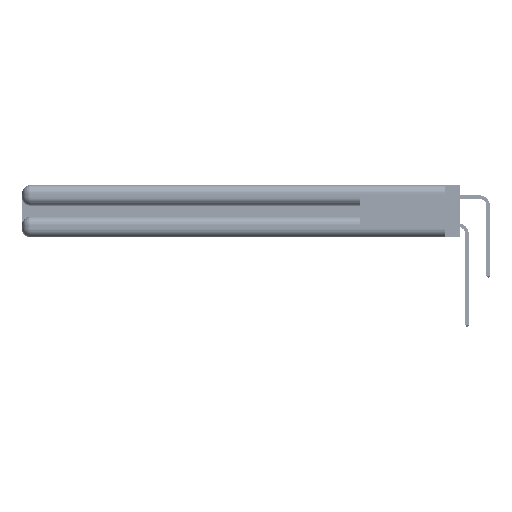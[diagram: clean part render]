
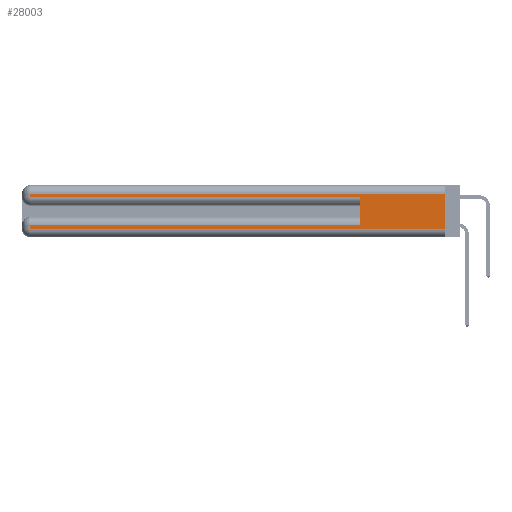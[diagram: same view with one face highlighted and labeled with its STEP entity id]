
A CAD part, left-side view. The second image highlights one B-rep face of the part: STEP entity #28003.
In plain terms, the highlighted planar face has unit normal (-1, 0, 0).
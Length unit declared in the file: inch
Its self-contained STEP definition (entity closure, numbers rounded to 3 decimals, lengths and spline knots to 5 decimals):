
#522 = CARTESIAN_POINT ( 'NONE',  ( 0., 0., 0.37 ) ) ;
#629 = CARTESIAN_POINT ( 'NONE',  ( 0., 0., 0.085 ) ) ;
#1703 = ORIENTED_EDGE ( 'NONE', *, *, #43113, .F. ) ;
#3313 = LINE ( 'NONE', #629, #13227 ) ;
#3759 = ORIENTED_EDGE ( 'NONE', *, *, #35805, .T. ) ;
#3783 = FACE_OUTER_BOUND ( 'NONE', #12405, .T. ) ;
#3843 = EDGE_CURVE ( 'NONE', #17330, #5140, #22326, .T. ) ;
#5140 = VERTEX_POINT ( 'NONE', #45637 ) ;
#5736 = ORIENTED_EDGE ( 'NONE', *, *, #45919, .T. ) ;
#9305 = PLANE ( 'NONE',  #9747 ) ;
#9747 = AXIS2_PLACEMENT_3D ( 'NONE', #522, #17726, #46899 ) ;
#9987 = CARTESIAN_POINT ( 'NONE',  ( 0., 2.94, 0.37 ) ) ;
#10115 = CARTESIAN_POINT ( 'NONE',  ( 0., 0., 0.285 ) ) ;
#11299 = VECTOR ( 'NONE', #47734, 39.37008 ) ;
#11415 = LINE ( 'NONE', #25395, #32263 ) ;
#11681 = EDGE_CURVE ( 'NONE', #12566, #37093, #11415, .T. ) ;
#12405 = EDGE_LOOP ( 'NONE', ( #1703, #5736, #18234, #43026, #13668, #35899, #3759, #41088 ) ) ;
#12566 = VERTEX_POINT ( 'NONE', #14197 ) ;
#13227 = VECTOR ( 'NONE', #34418, 39.37008 ) ;
#13397 = EDGE_CURVE ( 'NONE', #28808, #53611, #3313, .T. ) ;
#13668 = ORIENTED_EDGE ( 'NONE', *, *, #38563, .F. ) ;
#14197 = CARTESIAN_POINT ( 'NONE',  ( 0., 2.94, 0.06 ) ) ;
#14867 = CARTESIAN_POINT ( 'NONE',  ( 0., 2.94, 0.085 ) ) ;
#16920 = DIRECTION ( 'NONE',  ( 0., 0., 1. ) ) ;
#17330 = VERTEX_POINT ( 'NONE', #19297 ) ;
#17409 = VECTOR ( 'NONE', #16920, 39.37008 ) ;
#17726 = DIRECTION ( 'NONE',  ( 1., 0., 0. ) ) ;
#18234 = ORIENTED_EDGE ( 'NONE', *, *, #23566, .T. ) ;
#19297 = CARTESIAN_POINT ( 'NONE',  ( 0., 2.94, 0.285 ) ) ;
#22326 = LINE ( 'NONE', #10115, #52970 ) ;
#22356 = LINE ( 'NONE', #22564, #11299 ) ;
#22564 = CARTESIAN_POINT ( 'NONE',  ( 0., 0., 0.31 ) ) ;
#22972 = LINE ( 'NONE', #39058, #43829 ) ;
#23566 = EDGE_CURVE ( 'NONE', #33350, #17330, #24804, .T. ) ;
#24804 = LINE ( 'NONE', #9987, #26114 ) ;
#25395 = CARTESIAN_POINT ( 'NONE',  ( 0., 0., 0.06 ) ) ;
#26114 = VECTOR ( 'NONE', #39190, 39.37008 ) ;
#28003 = ADVANCED_FACE ( 'NONE', ( #3783 ), #9305, .F. ) ;
#28507 = LINE ( 'NONE', #46086, #17409 ) ;
#28808 = VERTEX_POINT ( 'NONE', #51543 ) ;
#29594 = DIRECTION ( 'NONE',  ( 0., -1., 0. ) ) ;
#30323 = CARTESIAN_POINT ( 'NONE',  ( 0., 2.94, 0.31 ) ) ;
#31305 = CARTESIAN_POINT ( 'NONE',  ( 0., 0., 0.06 ) ) ;
#32263 = VECTOR ( 'NONE', #29594, 39.37008 ) ;
#33282 = LINE ( 'NONE', #41391, #43045 ) ;
#33350 = VERTEX_POINT ( 'NONE', #30323 ) ;
#34418 = DIRECTION ( 'NONE',  ( 0., 1., 0. ) ) ;
#34880 = DIRECTION ( 'NONE',  ( 0., 0., -1. ) ) ;
#35805 = EDGE_CURVE ( 'NONE', #53611, #12566, #22972, .T. ) ;
#35899 = ORIENTED_EDGE ( 'NONE', *, *, #13397, .T. ) ;
#37093 = VERTEX_POINT ( 'NONE', #31305 ) ;
#38563 = EDGE_CURVE ( 'NONE', #28808, #5140, #28507, .T. ) ;
#39058 = CARTESIAN_POINT ( 'NONE',  ( 0., 2.94, 0.37 ) ) ;
#39190 = DIRECTION ( 'NONE',  ( 0., 0., -1. ) ) ;
#41088 = ORIENTED_EDGE ( 'NONE', *, *, #11681, .T. ) ;
#41391 = CARTESIAN_POINT ( 'NONE',  ( 0., 0., 0.37 ) ) ;
#43026 = ORIENTED_EDGE ( 'NONE', *, *, #3843, .T. ) ;
#43045 = VECTOR ( 'NONE', #45584, 39.37008 ) ;
#43113 = EDGE_CURVE ( 'NONE', #44246, #37093, #33282, .T. ) ;
#43494 = DIRECTION ( 'NONE',  ( 0., -1., 0. ) ) ;
#43829 = VECTOR ( 'NONE', #34880, 39.37008 ) ;
#44246 = VERTEX_POINT ( 'NONE', #53310 ) ;
#45584 = DIRECTION ( 'NONE',  ( 0., 0., -1. ) ) ;
#45637 = CARTESIAN_POINT ( 'NONE',  ( 0., 0.6, 0.285 ) ) ;
#45919 = EDGE_CURVE ( 'NONE', #44246, #33350, #22356, .T. ) ;
#46086 = CARTESIAN_POINT ( 'NONE',  ( 0., 0.6, 0.145 ) ) ;
#46899 = DIRECTION ( 'NONE',  ( 0., 0., -1. ) ) ;
#47734 = DIRECTION ( 'NONE',  ( 0., 1., 0. ) ) ;
#51543 = CARTESIAN_POINT ( 'NONE',  ( 0., 0.6, 0.085 ) ) ;
#52970 = VECTOR ( 'NONE', #43494, 39.37008 ) ;
#53310 = CARTESIAN_POINT ( 'NONE',  ( 0., 0., 0.31 ) ) ;
#53611 = VERTEX_POINT ( 'NONE', #14867 ) ;
